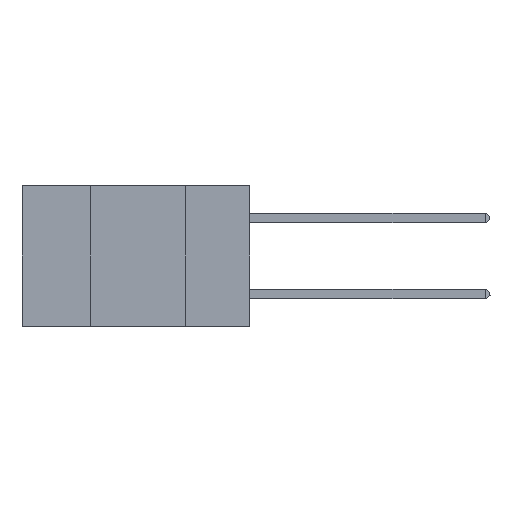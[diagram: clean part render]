
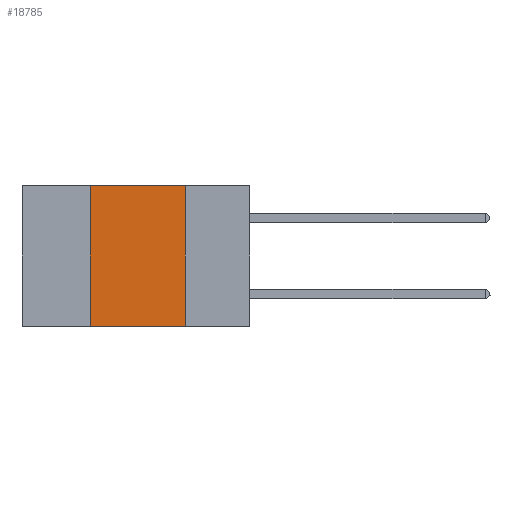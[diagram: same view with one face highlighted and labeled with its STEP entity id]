
A CAD part, left-side view. The second image highlights one B-rep face of the part: STEP entity #18785.
In plain terms, the highlighted planar face has unit normal (-1, 0, 0).
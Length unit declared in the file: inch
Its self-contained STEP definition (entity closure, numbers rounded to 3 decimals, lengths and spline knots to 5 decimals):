
#323 = DIRECTION ( 'NONE',  ( 0., 0., -1. ) ) ;
#852 = LINE ( 'NONE', #18534, #2710 ) ;
#1011 = VERTEX_POINT ( 'NONE', #20175 ) ;
#1105 = LINE ( 'NONE', #15351, #1611 ) ;
#1611 = VECTOR ( 'NONE', #3651, 39.37008 ) ;
#2206 = CARTESIAN_POINT ( 'NONE',  ( 0., 0.6, -0.37 ) ) ;
#2378 = ORIENTED_EDGE ( 'NONE', *, *, #13232, .F. ) ;
#2710 = VECTOR ( 'NONE', #18463, 39.37008 ) ;
#2837 = ORIENTED_EDGE ( 'NONE', *, *, #9196, .T. ) ;
#3651 = DIRECTION ( 'NONE',  ( 0., 0., -1. ) ) ;
#4027 = VERTEX_POINT ( 'NONE', #15267 ) ;
#5268 = ORIENTED_EDGE ( 'NONE', *, *, #8487, .F. ) ;
#5433 = CARTESIAN_POINT ( 'NONE',  ( 0., 0.6, 0. ) ) ;
#5661 = PLANE ( 'NONE',  #10343 ) ;
#7695 = LINE ( 'NONE', #7892, #11657 ) ;
#7892 = CARTESIAN_POINT ( 'NONE',  ( 0., 0.6, 0. ) ) ;
#7927 = FACE_OUTER_BOUND ( 'NONE', #20668, .T. ) ;
#8487 = EDGE_CURVE ( 'NONE', #16023, #4027, #7695, .T. ) ;
#8733 = CARTESIAN_POINT ( 'NONE',  ( 0., 0.42, -0.37 ) ) ;
#8848 = DIRECTION ( 'NONE',  ( 0., -1., 0. ) ) ;
#8966 = LINE ( 'NONE', #2206, #16875 ) ;
#9086 = DIRECTION ( 'NONE',  ( 1., 0., 0. ) ) ;
#9196 = EDGE_CURVE ( 'NONE', #15330, #1011, #8966, .T. ) ;
#10343 = AXIS2_PLACEMENT_3D ( 'NONE', #5433, #9086, #323 ) ;
#11657 = VECTOR ( 'NONE', #16227, 39.37008 ) ;
#12512 = EDGE_CURVE ( 'NONE', #15330, #16023, #852, .T. ) ;
#13232 = EDGE_CURVE ( 'NONE', #4027, #1011, #1105, .T. ) ;
#15267 = CARTESIAN_POINT ( 'NONE',  ( 0., 0.17, 0. ) ) ;
#15330 = VERTEX_POINT ( 'NONE', #8733 ) ;
#15351 = CARTESIAN_POINT ( 'NONE',  ( 0., 0.17, 0. ) ) ;
#16023 = VERTEX_POINT ( 'NONE', #16402 ) ;
#16227 = DIRECTION ( 'NONE',  ( 0., -1., 0. ) ) ;
#16402 = CARTESIAN_POINT ( 'NONE',  ( 0., 0.42, 0. ) ) ;
#16875 = VECTOR ( 'NONE', #8848, 39.37008 ) ;
#18463 = DIRECTION ( 'NONE',  ( 0., 0., 1. ) ) ;
#18534 = CARTESIAN_POINT ( 'NONE',  ( 0., 0.42, 0. ) ) ;
#18785 = ADVANCED_FACE ( 'NONE', ( #7927 ), #5661, .F. ) ;
#20089 = ORIENTED_EDGE ( 'NONE', *, *, #12512, .F. ) ;
#20175 = CARTESIAN_POINT ( 'NONE',  ( 0., 0.17, -0.37 ) ) ;
#20668 = EDGE_LOOP ( 'NONE', ( #2378, #5268, #20089, #2837 ) ) ;
